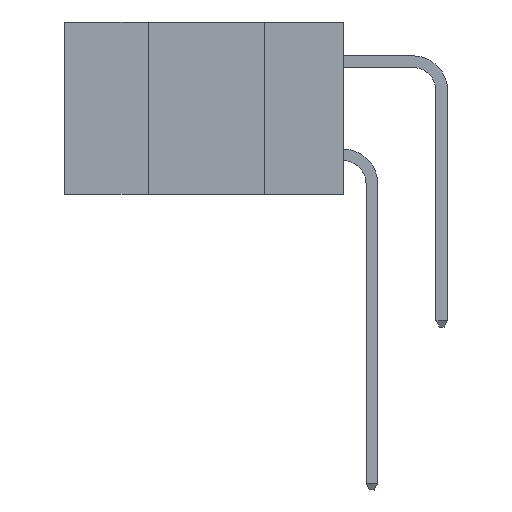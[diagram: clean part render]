
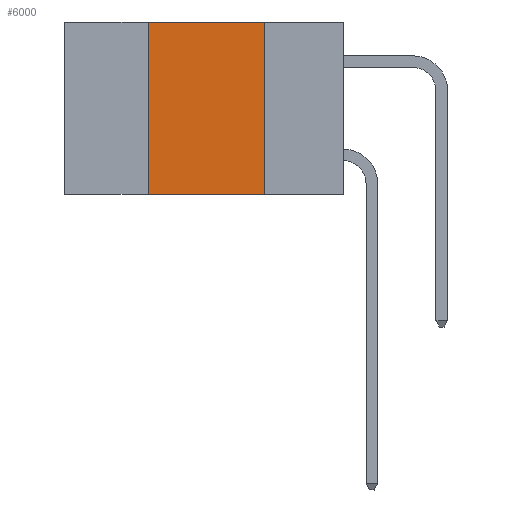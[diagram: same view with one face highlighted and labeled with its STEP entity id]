
A CAD part, left-side view. The second image highlights one B-rep face of the part: STEP entity #6000.
In plain terms, the highlighted planar face has unit normal (-1, 0, 0).
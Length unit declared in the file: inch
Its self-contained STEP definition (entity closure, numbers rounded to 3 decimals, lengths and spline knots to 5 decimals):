
#1659 = CARTESIAN_POINT ( 'NONE',  ( 0., 0.42, -0.37 ) ) ;
#2704 = DIRECTION ( 'NONE',  ( 1., 0., 0. ) ) ;
#3102 = CARTESIAN_POINT ( 'NONE',  ( 0., 0.42, 0. ) ) ;
#3372 = CARTESIAN_POINT ( 'NONE',  ( 0., 0.17, -0.37 ) ) ;
#3507 = ORIENTED_EDGE ( 'NONE', *, *, #7909, .F. ) ;
#4318 = DIRECTION ( 'NONE',  ( 0., -1., 0. ) ) ;
#5706 = EDGE_CURVE ( 'NONE', #16983, #24856, #15118, .T. ) ;
#5782 = VECTOR ( 'NONE', #4318, 39.37008 ) ;
#6000 = ADVANCED_FACE ( 'NONE', ( #20968 ), #13675, .F. ) ;
#6067 = CARTESIAN_POINT ( 'NONE',  ( 0., 0.6, -0.37 ) ) ;
#6123 = VECTOR ( 'NONE', #18155, 39.37008 ) ;
#6805 = LINE ( 'NONE', #27175, #6123 ) ;
#7909 = EDGE_CURVE ( 'NONE', #21343, #16983, #9055, .T. ) ;
#9055 = LINE ( 'NONE', #19317, #15645 ) ;
#10499 = DIRECTION ( 'NONE',  ( 0., 0., 1. ) ) ;
#11832 = CARTESIAN_POINT ( 'NONE',  ( 0., 0.6, 0. ) ) ;
#12910 = VERTEX_POINT ( 'NONE', #3372 ) ;
#13675 = PLANE ( 'NONE',  #23150 ) ;
#13694 = LINE ( 'NONE', #6067, #24049 ) ;
#14741 = ORIENTED_EDGE ( 'NONE', *, *, #5706, .F. ) ;
#15019 = CARTESIAN_POINT ( 'NONE',  ( 0., 0.6, 0. ) ) ;
#15118 = LINE ( 'NONE', #15019, #5782 ) ;
#15645 = VECTOR ( 'NONE', #10499, 39.37008 ) ;
#16487 = EDGE_CURVE ( 'NONE', #21343, #12910, #13694, .T. ) ;
#16983 = VERTEX_POINT ( 'NONE', #3102 ) ;
#18155 = DIRECTION ( 'NONE',  ( 0., 0., -1. ) ) ;
#19192 = CARTESIAN_POINT ( 'NONE',  ( 0., 0.17, 0. ) ) ;
#19317 = CARTESIAN_POINT ( 'NONE',  ( 0., 0.42, 0. ) ) ;
#20968 = FACE_OUTER_BOUND ( 'NONE', #27248, .T. ) ;
#21343 = VERTEX_POINT ( 'NONE', #1659 ) ;
#21540 = DIRECTION ( 'NONE',  ( 0., -1., 0. ) ) ;
#23150 = AXIS2_PLACEMENT_3D ( 'NONE', #11832, #2704, #27066 ) ;
#24027 = ORIENTED_EDGE ( 'NONE', *, *, #16487, .T. ) ;
#24049 = VECTOR ( 'NONE', #21540, 39.37008 ) ;
#24753 = EDGE_CURVE ( 'NONE', #24856, #12910, #6805, .T. ) ;
#24856 = VERTEX_POINT ( 'NONE', #19192 ) ;
#27066 = DIRECTION ( 'NONE',  ( 0., 0., -1. ) ) ;
#27146 = ORIENTED_EDGE ( 'NONE', *, *, #24753, .F. ) ;
#27175 = CARTESIAN_POINT ( 'NONE',  ( 0., 0.17, 0. ) ) ;
#27248 = EDGE_LOOP ( 'NONE', ( #27146, #14741, #3507, #24027 ) ) ;
